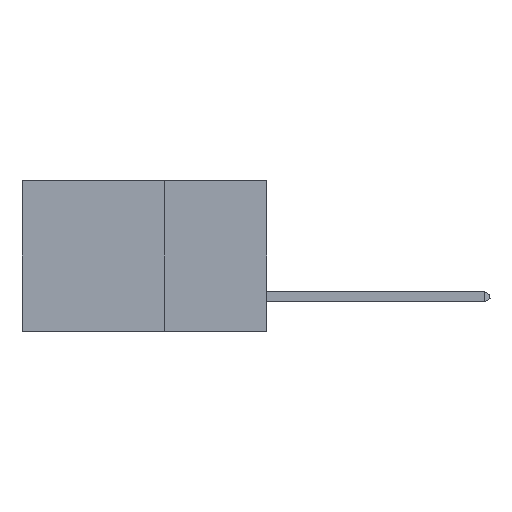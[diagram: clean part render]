
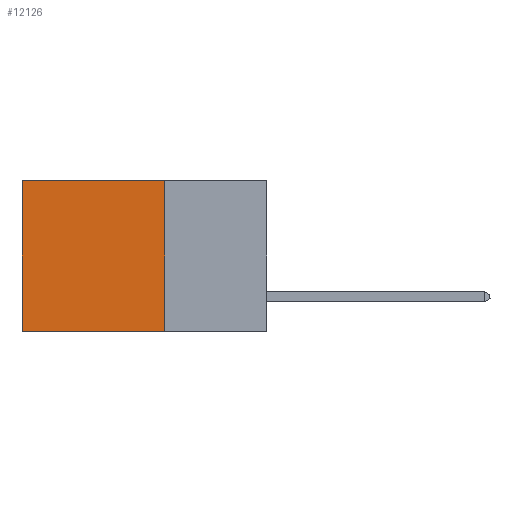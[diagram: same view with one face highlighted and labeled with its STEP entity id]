
A CAD part, left-side view. The second image highlights one B-rep face of the part: STEP entity #12126.
In plain terms, the highlighted planar face has unit normal (-1, 0, 0).
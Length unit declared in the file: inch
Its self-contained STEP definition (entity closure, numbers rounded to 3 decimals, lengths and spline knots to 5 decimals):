
#2167 = EDGE_CURVE ( 'NONE', #27100, #33757, #3770, .T. ) ;
#3770 = LINE ( 'NONE', #25037, #11676 ) ;
#4549 = LINE ( 'NONE', #21571, #17306 ) ;
#7397 = PLANE ( 'NONE',  #30943 ) ;
#10263 = EDGE_CURVE ( 'NONE', #17413, #33757, #27713, .T. ) ;
#11676 = VECTOR ( 'NONE', #22707, 39.37008 ) ;
#12126 = ADVANCED_FACE ( 'NONE', ( #27551 ), #7397, .F. ) ;
#12221 = CARTESIAN_POINT ( 'NONE',  ( 0.2875, 0.25, 0. ) ) ;
#13093 = VERTEX_POINT ( 'NONE', #12221 ) ;
#13185 = CARTESIAN_POINT ( 'NONE',  ( 0.2875, 0.6, -0.37 ) ) ;
#14164 = CARTESIAN_POINT ( 'NONE',  ( 0.2875, 0.25, -0.37 ) ) ;
#14757 = CARTESIAN_POINT ( 'NONE',  ( 0.2875, 0.25, -0.37 ) ) ;
#14819 = EDGE_CURVE ( 'NONE', #13093, #27100, #4549, .T. ) ;
#15446 = EDGE_CURVE ( 'NONE', #13093, #17413, #18130, .T. ) ;
#16250 = DIRECTION ( 'NONE',  ( 0., 1., 0. ) ) ;
#16780 = CARTESIAN_POINT ( 'NONE',  ( 0.2875, 0.6, 0. ) ) ;
#17306 = VECTOR ( 'NONE', #16250, 39.37008 ) ;
#17413 = VERTEX_POINT ( 'NONE', #14164 ) ;
#17429 = DIRECTION ( 'NONE',  ( 0., 1., 0. ) ) ;
#17769 = DIRECTION ( 'NONE',  ( 1., 0., 0. ) ) ;
#18130 = LINE ( 'NONE', #20827, #18483 ) ;
#18483 = VECTOR ( 'NONE', #26076, 39.37008 ) ;
#18989 = VECTOR ( 'NONE', #17429, 39.37008 ) ;
#20415 = DIRECTION ( 'NONE',  ( 0., 0., -1. ) ) ;
#20807 = ORIENTED_EDGE ( 'NONE', *, *, #15446, .F. ) ;
#20827 = CARTESIAN_POINT ( 'NONE',  ( 0.2875, 0.25, 0. ) ) ;
#21571 = CARTESIAN_POINT ( 'NONE',  ( 0.2875, 0.25, 0. ) ) ;
#22320 = ORIENTED_EDGE ( 'NONE', *, *, #14819, .T. ) ;
#22707 = DIRECTION ( 'NONE',  ( 0., 0., -1. ) ) ;
#25037 = CARTESIAN_POINT ( 'NONE',  ( 0.2875, 0.6, 0. ) ) ;
#26076 = DIRECTION ( 'NONE',  ( 0., 0., -1. ) ) ;
#27100 = VERTEX_POINT ( 'NONE', #16780 ) ;
#27551 = FACE_OUTER_BOUND ( 'NONE', #30963, .T. ) ;
#27713 = LINE ( 'NONE', #14757, #18989 ) ;
#30943 = AXIS2_PLACEMENT_3D ( 'NONE', #33523, #17769, #20415 ) ;
#30963 = EDGE_LOOP ( 'NONE', ( #31368, #32616, #20807, #22320 ) ) ;
#31368 = ORIENTED_EDGE ( 'NONE', *, *, #2167, .T. ) ;
#32616 = ORIENTED_EDGE ( 'NONE', *, *, #10263, .F. ) ;
#33523 = CARTESIAN_POINT ( 'NONE',  ( 0.2875, 0.25, 0. ) ) ;
#33757 = VERTEX_POINT ( 'NONE', #13185 ) ;
